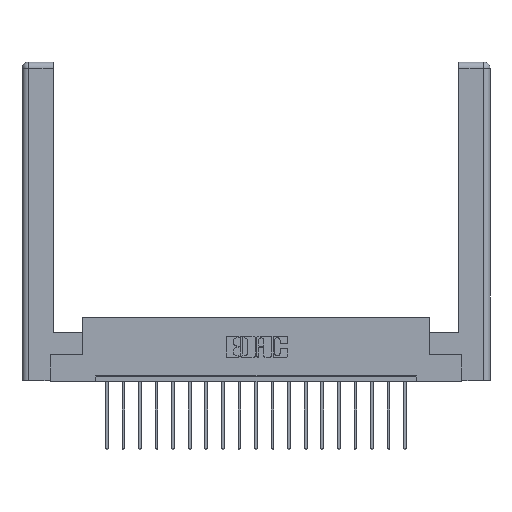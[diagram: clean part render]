
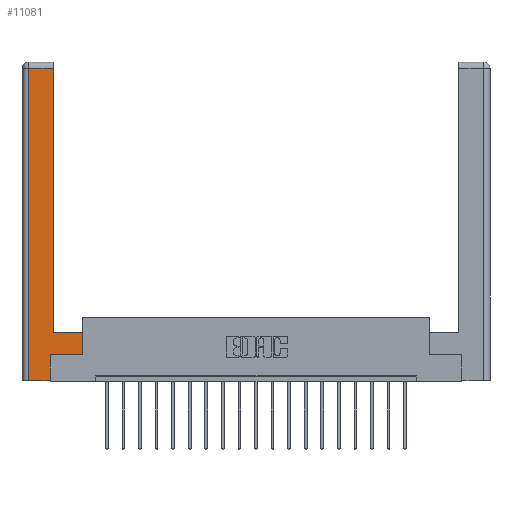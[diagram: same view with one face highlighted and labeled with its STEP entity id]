
A CAD part, top view. The second image highlights one B-rep face of the part: STEP entity #11081.
In plain terms, the highlighted planar face has unit normal (0, 0, 1).
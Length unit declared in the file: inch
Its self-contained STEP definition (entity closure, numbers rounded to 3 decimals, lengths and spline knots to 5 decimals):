
#159 = LINE ( 'NONE', #19510, #15891 ) ;
#501 = CARTESIAN_POINT ( 'NONE',  ( 0.565, 0.45, 0. ) ) ;
#880 = VERTEX_POINT ( 'NONE', #3326 ) ;
#1090 = VECTOR ( 'NONE', #10985, 39.37008 ) ;
#1317 = VECTOR ( 'NONE', #12170, 39.37008 ) ;
#1334 = CARTESIAN_POINT ( 'NONE',  ( 0.265, 0., 0. ) ) ;
#1343 = EDGE_LOOP ( 'NONE', ( #5582, #6938, #16632, #18158, #14736, #13343, #11845, #9953 ) ) ;
#3326 = CARTESIAN_POINT ( 'NONE',  ( 0.0615, 0., 0. ) ) ;
#3424 = LINE ( 'NONE', #5731, #19194 ) ;
#3614 = DIRECTION ( 'NONE',  ( 0., 1., 0. ) ) ;
#4643 = PLANE ( 'NONE',  #9151 ) ;
#5052 = EDGE_CURVE ( 'NONE', #7363, #880, #159, .T. ) ;
#5307 = EDGE_CURVE ( 'NONE', #14027, #6012, #10374, .T. ) ;
#5582 = ORIENTED_EDGE ( 'NONE', *, *, #5307, .T. ) ;
#5731 = CARTESIAN_POINT ( 'NONE',  ( 0.565, 0.245, 0. ) ) ;
#5972 = LINE ( 'NONE', #10976, #18644 ) ;
#6012 = VERTEX_POINT ( 'NONE', #17813 ) ;
#6278 = DIRECTION ( 'NONE',  ( -1., 0., 0. ) ) ;
#6296 = CARTESIAN_POINT ( 'NONE',  ( 0.295, 0.45, 0. ) ) ;
#6938 = ORIENTED_EDGE ( 'NONE', *, *, #19737, .T. ) ;
#7363 = VERTEX_POINT ( 'NONE', #12960 ) ;
#7511 = DIRECTION ( 'NONE',  ( 1., 0., 0. ) ) ;
#7917 = EDGE_CURVE ( 'NONE', #880, #10759, #12304, .T. ) ;
#8101 = CARTESIAN_POINT ( 'NONE',  ( 0.295, 0.45, 0. ) ) ;
#8250 = VECTOR ( 'NONE', #18443, 39.37008 ) ;
#8869 = VERTEX_POINT ( 'NONE', #16530 ) ;
#9151 = AXIS2_PLACEMENT_3D ( 'NONE', #10944, #16870, #18334 ) ;
#9623 = FACE_OUTER_BOUND ( 'NONE', #1343, .T. ) ;
#9953 = ORIENTED_EDGE ( 'NONE', *, *, #14967, .T. ) ;
#10374 = LINE ( 'NONE', #18648, #1090 ) ;
#10658 = EDGE_CURVE ( 'NONE', #19746, #8869, #3424, .T. ) ;
#10759 = VERTEX_POINT ( 'NONE', #1334 ) ;
#10944 = CARTESIAN_POINT ( 'NONE',  ( 0., 0., 0. ) ) ;
#10976 = CARTESIAN_POINT ( 'NONE',  ( 0.0615, 2.94, 0. ) ) ;
#10985 = DIRECTION ( 'NONE',  ( 0., 1., 0. ) ) ;
#11081 = ADVANCED_FACE ( 'NONE', ( #9623 ), #4643, .F. ) ;
#11367 = LINE ( 'NONE', #6296, #8250 ) ;
#11562 = EDGE_CURVE ( 'NONE', #8869, #17709, #14872, .T. ) ;
#11845 = ORIENTED_EDGE ( 'NONE', *, *, #11562, .T. ) ;
#12026 = VECTOR ( 'NONE', #3614, 39.37008 ) ;
#12170 = DIRECTION ( 'NONE',  ( 1., 0., 0. ) ) ;
#12304 = LINE ( 'NONE', #16928, #1317 ) ;
#12960 = CARTESIAN_POINT ( 'NONE',  ( 0.0615, 2.94, 0. ) ) ;
#13343 = ORIENTED_EDGE ( 'NONE', *, *, #10658, .T. ) ;
#14027 = VERTEX_POINT ( 'NONE', #8101 ) ;
#14248 = DIRECTION ( 'NONE',  ( 0., 1., 0. ) ) ;
#14736 = ORIENTED_EDGE ( 'NONE', *, *, #16366, .T. ) ;
#14872 = LINE ( 'NONE', #501, #18461 ) ;
#14967 = EDGE_CURVE ( 'NONE', #17709, #14027, #11367, .T. ) ;
#15151 = CARTESIAN_POINT ( 'NONE',  ( 0.565, 0.45, 0. ) ) ;
#15891 = VECTOR ( 'NONE', #16655, 39.37008 ) ;
#16327 = LINE ( 'NONE', #17461, #12026 ) ;
#16366 = EDGE_CURVE ( 'NONE', #10759, #19746, #16327, .T. ) ;
#16530 = CARTESIAN_POINT ( 'NONE',  ( 0.565, 0.245, 0. ) ) ;
#16632 = ORIENTED_EDGE ( 'NONE', *, *, #5052, .T. ) ;
#16655 = DIRECTION ( 'NONE',  ( 0., -1., 0. ) ) ;
#16870 = DIRECTION ( 'NONE',  ( 0., 0., -1. ) ) ;
#16928 = CARTESIAN_POINT ( 'NONE',  ( 0.265, 0., 0. ) ) ;
#17051 = CARTESIAN_POINT ( 'NONE',  ( 0.265, 0.245, 0. ) ) ;
#17461 = CARTESIAN_POINT ( 'NONE',  ( 0.265, 0.245, 0. ) ) ;
#17709 = VERTEX_POINT ( 'NONE', #15151 ) ;
#17813 = CARTESIAN_POINT ( 'NONE',  ( 0.295, 2.94, 0. ) ) ;
#18158 = ORIENTED_EDGE ( 'NONE', *, *, #7917, .T. ) ;
#18334 = DIRECTION ( 'NONE',  ( -1., 0., 0. ) ) ;
#18443 = DIRECTION ( 'NONE',  ( -1., 0., 0. ) ) ;
#18461 = VECTOR ( 'NONE', #14248, 39.37008 ) ;
#18644 = VECTOR ( 'NONE', #6278, 39.37008 ) ;
#18648 = CARTESIAN_POINT ( 'NONE',  ( 0.295, 3., 0. ) ) ;
#19194 = VECTOR ( 'NONE', #7511, 39.37008 ) ;
#19510 = CARTESIAN_POINT ( 'NONE',  ( 0.0615, 0., 0. ) ) ;
#19737 = EDGE_CURVE ( 'NONE', #6012, #7363, #5972, .T. ) ;
#19746 = VERTEX_POINT ( 'NONE', #17051 ) ;
